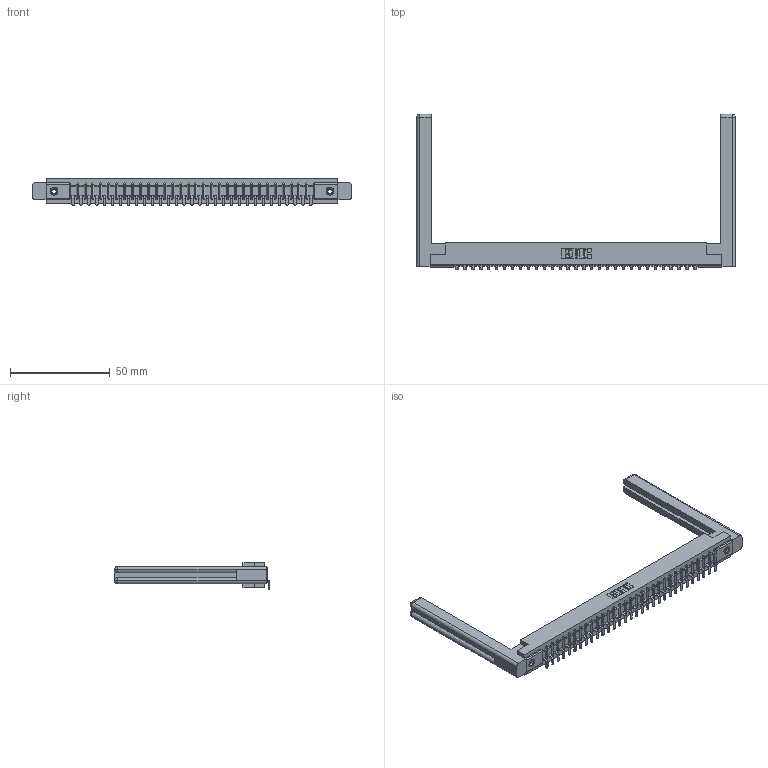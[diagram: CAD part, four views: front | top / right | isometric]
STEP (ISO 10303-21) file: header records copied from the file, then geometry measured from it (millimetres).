
FILE_DESCRIPTION (( 'STEP AP203' ), '1' );
FILE_NAME ('307-031-453-158.STEP', '2020-09-28T14:26:14', ( '' ), ( '' ), 'SwSTEP 2.0', 'SolidWorks 2020', '' );
FILE_SCHEMA (( 'CONFIG_CONTROL_DESIGN' ));
Length unit declared in the file: inch
Products named in the file (5): 307-290-002_553; 307-220-058; 307 Part_.156 Dia Mounting Holes; 307-031-453-158; 345-250-001_345-250-001-102
Assembly tree (36 placements, depth 2):
  307-031-453-158
    307 Part_.156 Dia Mounting Holes
    307-290-002_553  x31
    307-220-058  x2
    345-250-001_345-250-001-102  x2
Bounding box: 159.46 x 77.64 x 13.5 mm (x, y, z)
Volume: 24102.4 mm3; surface area: 25938.6 mm2
Topology: 36 solids, 36 shells, 2710 faces, 8241 edges, 5394 vertices
Faces by surface type: plane 1611, cylinder 1011, sphere 64, torus 12, cone 12
Entity records: 31419 total; most frequent: CARTESIAN_POINT 5307, ORIENTED_EDGE 5236, DIRECTION 5122, EDGE_CURVE 2618, VECTOR 1996, LINE 1996, VERTEX_POINT 1694, AXIS2_PLACEMENT_3D 1563
